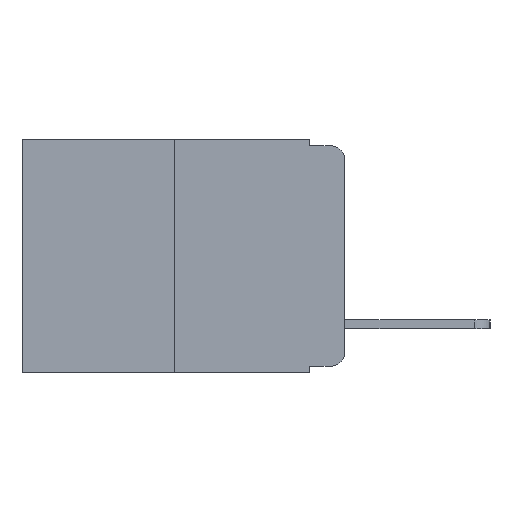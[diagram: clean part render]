
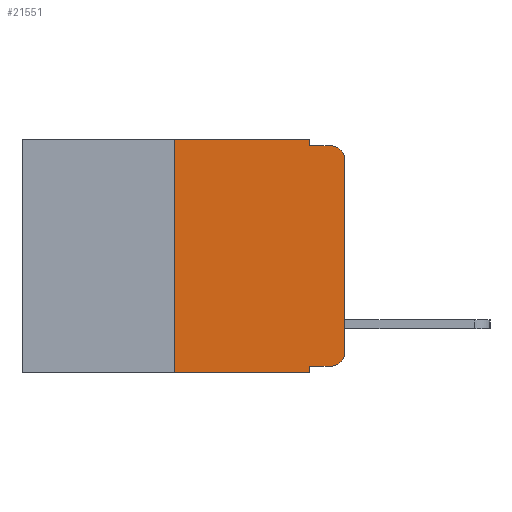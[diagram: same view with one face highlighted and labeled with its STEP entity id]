
A CAD part, left-side view. The second image highlights one B-rep face of the part: STEP entity #21551.
In plain terms, the highlighted planar face has unit normal (-1, 0, 0).
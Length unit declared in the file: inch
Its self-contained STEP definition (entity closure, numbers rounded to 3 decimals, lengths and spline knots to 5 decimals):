
#306 = CARTESIAN_POINT ( 'NONE',  ( 0., 0.02, -0.313 ) ) ;
#339 = CARTESIAN_POINT ( 'NONE',  ( 0., 0.051, 0. ) ) ;
#344 = EDGE_CURVE ( 'NONE', #19565, #5344, #3515, .T. ) ;
#1353 = VECTOR ( 'NONE', #19761, 39.37008 ) ;
#1382 = DIRECTION ( 'NONE',  ( 0., 0., -1. ) ) ;
#2266 = DIRECTION ( 'NONE',  ( 0., 0., -1. ) ) ;
#2564 = VERTEX_POINT ( 'NONE', #8737 ) ;
#2627 = LINE ( 'NONE', #18007, #22283 ) ;
#2715 = DIRECTION ( 'NONE',  ( -1., 0., 0. ) ) ;
#2855 = VECTOR ( 'NONE', #8014, 39.37008 ) ;
#2909 = CARTESIAN_POINT ( 'NONE',  ( 0., 0.051, 0. ) ) ;
#2983 = EDGE_CURVE ( 'NONE', #5344, #22653, #12782, .T. ) ;
#3515 = LINE ( 'NONE', #2909, #23120 ) ;
#3814 = FACE_OUTER_BOUND ( 'NONE', #23108, .T. ) ;
#3859 = LINE ( 'NONE', #339, #13425 ) ;
#3917 = CARTESIAN_POINT ( 'NONE',  ( 0., 0.25, 0. ) ) ;
#3997 = DIRECTION ( 'NONE',  ( 0., 0., 1. ) ) ;
#4003 = ORIENTED_EDGE ( 'NONE', *, *, #18771, .T. ) ;
#4273 = EDGE_CURVE ( 'NONE', #23657, #22653, #12108, .T. ) ;
#4357 = CARTESIAN_POINT ( 'NONE',  ( 0., 0.473, 0. ) ) ;
#4491 = VERTEX_POINT ( 'NONE', #5338 ) ;
#5338 = CARTESIAN_POINT ( 'NONE',  ( 0., 0.25, -0.343 ) ) ;
#5344 = VERTEX_POINT ( 'NONE', #10215 ) ;
#5576 = EDGE_CURVE ( 'NONE', #13349, #23657, #12642, .T. ) ;
#5816 = ORIENTED_EDGE ( 'NONE', *, *, #5576, .T. ) ;
#6122 = ORIENTED_EDGE ( 'NONE', *, *, #18171, .F. ) ;
#6465 = AXIS2_PLACEMENT_3D ( 'NONE', #306, #13770, #2266 ) ;
#6658 = CARTESIAN_POINT ( 'NONE',  ( 0., 0.051, 0. ) ) ;
#6814 = DIRECTION ( 'NONE',  ( 0., 0., -1. ) ) ;
#7604 = ORIENTED_EDGE ( 'NONE', *, *, #2983, .F. ) ;
#8014 = DIRECTION ( 'NONE',  ( 0., -1., 0. ) ) ;
#8737 = CARTESIAN_POINT ( 'NONE',  ( 0., 0.051, -0.343 ) ) ;
#9980 = VERTEX_POINT ( 'NONE', #11409 ) ;
#10215 = CARTESIAN_POINT ( 'NONE',  ( 0., 0.051, -0.01 ) ) ;
#10260 = LINE ( 'NONE', #3917, #19753 ) ;
#10446 = DIRECTION ( 'NONE',  ( 0., -1., 0. ) ) ;
#11409 = CARTESIAN_POINT ( 'NONE',  ( 0., 0.02, -0.333 ) ) ;
#11842 = CARTESIAN_POINT ( 'NONE',  ( 0., 0.051, -0.333 ) ) ;
#12108 = CIRCLE ( 'NONE', #20242, 0.02 ) ;
#12366 = ORIENTED_EDGE ( 'NONE', *, *, #23868, .F. ) ;
#12642 = LINE ( 'NONE', #24143, #22111 ) ;
#12782 = LINE ( 'NONE', #15960, #1353 ) ;
#12892 = DIRECTION ( 'NONE',  ( 1., 0., 0. ) ) ;
#13040 = VECTOR ( 'NONE', #21404, 39.37008 ) ;
#13349 = VERTEX_POINT ( 'NONE', #13846 ) ;
#13425 = VECTOR ( 'NONE', #17571, 39.37008 ) ;
#13770 = DIRECTION ( 'NONE',  ( -1., 0., 0. ) ) ;
#13846 = CARTESIAN_POINT ( 'NONE',  ( 0., 0., -0.313 ) ) ;
#14188 = CARTESIAN_POINT ( 'NONE',  ( 0., 0.02, -0.03 ) ) ;
#14713 = DIRECTION ( 'NONE',  ( 0., 0., 1. ) ) ;
#14758 = ORIENTED_EDGE ( 'NONE', *, *, #17494, .T. ) ;
#14761 = VERTEX_POINT ( 'NONE', #21859 ) ;
#15951 = VERTEX_POINT ( 'NONE', #16361 ) ;
#15960 = CARTESIAN_POINT ( 'NONE',  ( 0., 0.051, -0.01 ) ) ;
#16079 = DIRECTION ( 'NONE',  ( 0., 0., -1. ) ) ;
#16361 = CARTESIAN_POINT ( 'NONE',  ( 0., 0.25, 0. ) ) ;
#16500 = ORIENTED_EDGE ( 'NONE', *, *, #4273, .T. ) ;
#16556 = EDGE_CURVE ( 'NONE', #4491, #2564, #2627, .T. ) ;
#16601 = CIRCLE ( 'NONE', #6465, 0.02 ) ;
#17453 = LINE ( 'NONE', #4357, #13040 ) ;
#17461 = LINE ( 'NONE', #11842, #2855 ) ;
#17494 = EDGE_CURVE ( 'NONE', #9980, #13349, #16601, .T. ) ;
#17571 = DIRECTION ( 'NONE',  ( 0., 0., -1. ) ) ;
#17680 = ORIENTED_EDGE ( 'NONE', *, *, #344, .F. ) ;
#18007 = CARTESIAN_POINT ( 'NONE',  ( 0., 0.473, -0.343 ) ) ;
#18171 = EDGE_CURVE ( 'NONE', #15951, #19565, #17453, .T. ) ;
#18771 = EDGE_CURVE ( 'NONE', #14761, #9980, #17461, .T. ) ;
#19565 = VERTEX_POINT ( 'NONE', #6658 ) ;
#19753 = VECTOR ( 'NONE', #3997, 39.37008 ) ;
#19761 = DIRECTION ( 'NONE',  ( 0., -1., 0. ) ) ;
#20045 = EDGE_CURVE ( 'NONE', #14761, #2564, #3859, .T. ) ;
#20242 = AXIS2_PLACEMENT_3D ( 'NONE', #14188, #2715, #16079 ) ;
#21404 = DIRECTION ( 'NONE',  ( 0., -1., 0. ) ) ;
#21551 = ADVANCED_FACE ( 'NONE', ( #3814 ), #22316, .F. ) ;
#21859 = CARTESIAN_POINT ( 'NONE',  ( 0., 0.051, -0.333 ) ) ;
#22111 = VECTOR ( 'NONE', #14713, 39.37008 ) ;
#22283 = VECTOR ( 'NONE', #10446, 39.37008 ) ;
#22316 = PLANE ( 'NONE',  #23541 ) ;
#22653 = VERTEX_POINT ( 'NONE', #22823 ) ;
#22823 = CARTESIAN_POINT ( 'NONE',  ( 0., 0.02, -0.01 ) ) ;
#23013 = ORIENTED_EDGE ( 'NONE', *, *, #16556, .T. ) ;
#23108 = EDGE_LOOP ( 'NONE', ( #5816, #16500, #7604, #17680, #6122, #12366, #23013, #23628, #4003, #14758 ) ) ;
#23120 = VECTOR ( 'NONE', #6814, 39.37008 ) ;
#23541 = AXIS2_PLACEMENT_3D ( 'NONE', #24225, #12892, #1382 ) ;
#23628 = ORIENTED_EDGE ( 'NONE', *, *, #20045, .F. ) ;
#23657 = VERTEX_POINT ( 'NONE', #24203 ) ;
#23868 = EDGE_CURVE ( 'NONE', #4491, #15951, #10260, .T. ) ;
#24143 = CARTESIAN_POINT ( 'NONE',  ( 0., 0., 0. ) ) ;
#24203 = CARTESIAN_POINT ( 'NONE',  ( 0., 0., -0.03 ) ) ;
#24225 = CARTESIAN_POINT ( 'NONE',  ( 0., 0.473, 0. ) ) ;
